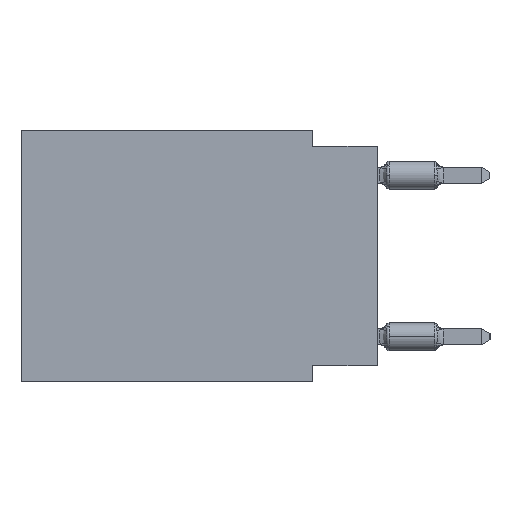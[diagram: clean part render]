
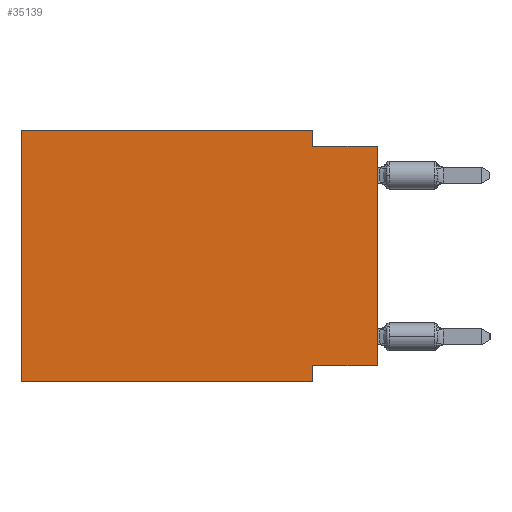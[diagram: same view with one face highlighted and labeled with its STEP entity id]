
A CAD part, left-side view. The second image highlights one B-rep face of the part: STEP entity #35139.
In plain terms, the highlighted planar face has unit normal (-1, 0, 0).
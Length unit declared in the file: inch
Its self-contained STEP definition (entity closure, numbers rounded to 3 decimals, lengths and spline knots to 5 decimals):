
#12 = VECTOR ( 'NONE', #8557, 39.37008 ) ;
#1319 = LINE ( 'NONE', #19158, #29124 ) ;
#2339 = ORIENTED_EDGE ( 'NONE', *, *, #53393, .F. ) ;
#3961 = PLANE ( 'NONE',  #16244 ) ;
#3973 = EDGE_CURVE ( 'NONE', #14993, #34749, #51754, .T. ) ;
#6214 = VECTOR ( 'NONE', #16055, 39.37008 ) ;
#6305 = LINE ( 'NONE', #54022, #55750 ) ;
#7108 = EDGE_CURVE ( 'NONE', #25235, #30890, #6305, .T. ) ;
#7680 = DIRECTION ( 'NONE',  ( 0., -1., 0. ) ) ;
#8157 = ORIENTED_EDGE ( 'NONE', *, *, #31080, .F. ) ;
#8557 = DIRECTION ( 'NONE',  ( 0., 0., -1. ) ) ;
#11111 = VERTEX_POINT ( 'NONE', #45839 ) ;
#12935 = VERTEX_POINT ( 'NONE', #35249 ) ;
#14993 = VERTEX_POINT ( 'NONE', #18556 ) ;
#15838 = ORIENTED_EDGE ( 'NONE', *, *, #20035, .T. ) ;
#15956 = DIRECTION ( 'NONE',  ( 0., -1., 0. ) ) ;
#16055 = DIRECTION ( 'NONE',  ( 0., -1., 0. ) ) ;
#16244 = AXIS2_PLACEMENT_3D ( 'NONE', #57793, #39370, #25908 ) ;
#16258 = VECTOR ( 'NONE', #7680, 39.37008 ) ;
#17993 = FACE_OUTER_BOUND ( 'NONE', #18139, .T. ) ;
#18139 = EDGE_LOOP ( 'NONE', ( #29502, #50097, #8157, #23027, #2339, #15838, #19700, #25529 ) ) ;
#18556 = CARTESIAN_POINT ( 'NONE',  ( 0., 0.1, -0.025 ) ) ;
#19158 = CARTESIAN_POINT ( 'NONE',  ( 0., 0., 0. ) ) ;
#19700 = ORIENTED_EDGE ( 'NONE', *, *, #29364, .F. ) ;
#19833 = CARTESIAN_POINT ( 'NONE',  ( 0., 0.55, -0.39 ) ) ;
#19929 = CARTESIAN_POINT ( 'NONE',  ( 0., 0.1, -0.39 ) ) ;
#20035 = EDGE_CURVE ( 'NONE', #51693, #23281, #24732, .T. ) ;
#20341 = CARTESIAN_POINT ( 'NONE',  ( 0., 0.55, -0.39 ) ) ;
#23027 = ORIENTED_EDGE ( 'NONE', *, *, #53996, .F. ) ;
#23281 = VERTEX_POINT ( 'NONE', #19929 ) ;
#24732 = LINE ( 'NONE', #20341, #56616 ) ;
#25235 = VERTEX_POINT ( 'NONE', #31958 ) ;
#25529 = ORIENTED_EDGE ( 'NONE', *, *, #7108, .F. ) ;
#25908 = DIRECTION ( 'NONE',  ( 0., 0., -1. ) ) ;
#28249 = LINE ( 'NONE', #54886, #29787 ) ;
#29124 = VECTOR ( 'NONE', #36449, 39.37008 ) ;
#29364 = EDGE_CURVE ( 'NONE', #30890, #23281, #28249, .T. ) ;
#29502 = ORIENTED_EDGE ( 'NONE', *, *, #32634, .T. ) ;
#29787 = VECTOR ( 'NONE', #32674, 39.37008 ) ;
#29935 = LINE ( 'NONE', #56547, #16258 ) ;
#30890 = VERTEX_POINT ( 'NONE', #37273 ) ;
#31080 = EDGE_CURVE ( 'NONE', #11111, #14993, #48637, .T. ) ;
#31958 = CARTESIAN_POINT ( 'NONE',  ( 0., 0., -0.365 ) ) ;
#32634 = EDGE_CURVE ( 'NONE', #25235, #34749, #1319, .T. ) ;
#32674 = DIRECTION ( 'NONE',  ( 0., 0., -1. ) ) ;
#32949 = DIRECTION ( 'NONE',  ( 0., 1., 0. ) ) ;
#34609 = CARTESIAN_POINT ( 'NONE',  ( 0., 0.1, 0. ) ) ;
#34749 = VERTEX_POINT ( 'NONE', #50922 ) ;
#35139 = ADVANCED_FACE ( 'NONE', ( #17993 ), #3961, .F. ) ;
#35249 = CARTESIAN_POINT ( 'NONE',  ( 0., 0.55, 0. ) ) ;
#35417 = DIRECTION ( 'NONE',  ( 0., 0., 1. ) ) ;
#36449 = DIRECTION ( 'NONE',  ( 0., 0., 1. ) ) ;
#37273 = CARTESIAN_POINT ( 'NONE',  ( 0., 0.1, -0.365 ) ) ;
#39370 = DIRECTION ( 'NONE',  ( 1., 0., 0. ) ) ;
#40652 = CARTESIAN_POINT ( 'NONE',  ( 0., 0.55, 0. ) ) ;
#45173 = VECTOR ( 'NONE', #35417, 39.37008 ) ;
#45839 = CARTESIAN_POINT ( 'NONE',  ( 0., 0.1, 0. ) ) ;
#47934 = CARTESIAN_POINT ( 'NONE',  ( 0., 0., -0.025 ) ) ;
#48637 = LINE ( 'NONE', #34609, #12 ) ;
#49714 = LINE ( 'NONE', #40652, #45173 ) ;
#50097 = ORIENTED_EDGE ( 'NONE', *, *, #3973, .F. ) ;
#50922 = CARTESIAN_POINT ( 'NONE',  ( 0., 0., -0.025 ) ) ;
#51693 = VERTEX_POINT ( 'NONE', #19833 ) ;
#51754 = LINE ( 'NONE', #47934, #6214 ) ;
#53393 = EDGE_CURVE ( 'NONE', #51693, #12935, #49714, .T. ) ;
#53996 = EDGE_CURVE ( 'NONE', #12935, #11111, #29935, .T. ) ;
#54022 = CARTESIAN_POINT ( 'NONE',  ( 0., 0., -0.365 ) ) ;
#54886 = CARTESIAN_POINT ( 'NONE',  ( 0., 0.1, -0.39 ) ) ;
#55750 = VECTOR ( 'NONE', #32949, 39.37008 ) ;
#56547 = CARTESIAN_POINT ( 'NONE',  ( 0., 0.55, 0. ) ) ;
#56616 = VECTOR ( 'NONE', #15956, 39.37008 ) ;
#57793 = CARTESIAN_POINT ( 'NONE',  ( 0., 0.55, 0. ) ) ;
